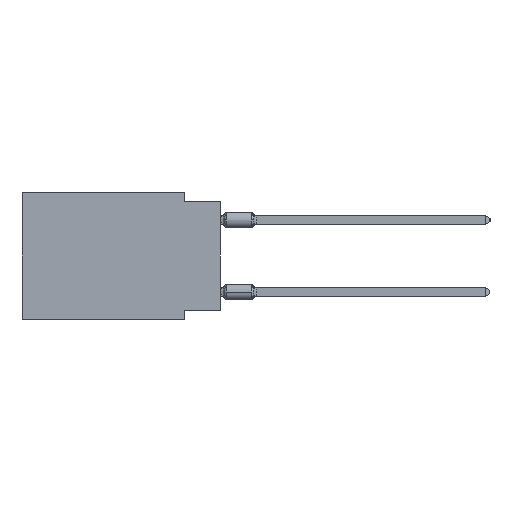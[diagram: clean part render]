
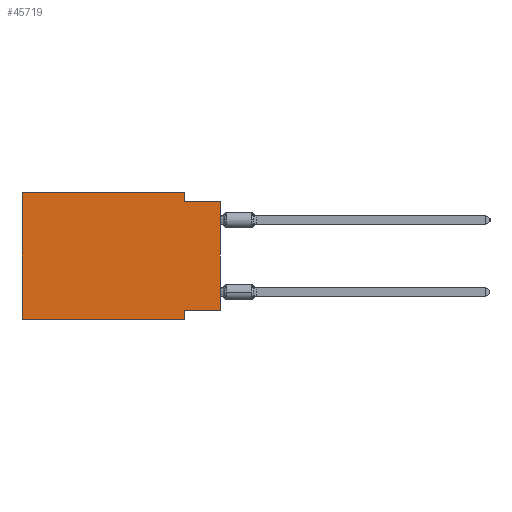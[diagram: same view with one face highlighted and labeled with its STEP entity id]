
A CAD part, left-side view. The second image highlights one B-rep face of the part: STEP entity #45719.
In plain terms, the highlighted planar face has unit normal (-1, 0, 0).
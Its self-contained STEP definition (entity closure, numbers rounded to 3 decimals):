
#1503 = CARTESIAN_POINT ( 'NONE',  ( 0., 13.97, -8.89 ) ) ;
#2421 = CARTESIAN_POINT ( 'NONE',  ( 0., 13.97, -8.89 ) ) ;
#2617 = CARTESIAN_POINT ( 'NONE',  ( 0., 2.54, 0. ) ) ;
#5274 = CARTESIAN_POINT ( 'NONE',  ( 0., 0., 0. ) ) ;
#5318 = VERTEX_POINT ( 'NONE', #34277 ) ;
#6966 = ORIENTED_EDGE ( 'NONE', *, *, #13096, .F. ) ;
#6985 = VECTOR ( 'NONE', #33532, 1000. ) ;
#7600 = DIRECTION ( 'NONE',  ( 0., 0., -1. ) ) ;
#7608 = LINE ( 'NONE', #27899, #28563 ) ;
#8690 = ORIENTED_EDGE ( 'NONE', *, *, #14452, .F. ) ;
#9925 = DIRECTION ( 'NONE',  ( 0., -1., 0. ) ) ;
#11632 = CARTESIAN_POINT ( 'NONE',  ( 0., 0., -8.255 ) ) ;
#12003 = CARTESIAN_POINT ( 'NONE',  ( 0., 13.97, 0. ) ) ;
#12917 = VERTEX_POINT ( 'NONE', #30679 ) ;
#13096 = EDGE_CURVE ( 'NONE', #50201, #5318, #27880, .T. ) ;
#13294 = EDGE_CURVE ( 'NONE', #20898, #40234, #38496, .T. ) ;
#13916 = ORIENTED_EDGE ( 'NONE', *, *, #34729, .T. ) ;
#14452 = EDGE_CURVE ( 'NONE', #28546, #12917, #22585, .T. ) ;
#15229 = VECTOR ( 'NONE', #26466, 1000. ) ;
#15240 = DIRECTION ( 'NONE',  ( 0., 0., 1. ) ) ;
#15717 = CARTESIAN_POINT ( 'NONE',  ( 0., 0., -0.635 ) ) ;
#20339 = EDGE_CURVE ( 'NONE', #20898, #51565, #46730, .T. ) ;
#20396 = CARTESIAN_POINT ( 'NONE',  ( 0., 0., -0.635 ) ) ;
#20777 = EDGE_CURVE ( 'NONE', #12917, #61230, #25393, .T. ) ;
#20898 = VERTEX_POINT ( 'NONE', #2421 ) ;
#21700 = CARTESIAN_POINT ( 'NONE',  ( 0., 2.54, -8.89 ) ) ;
#21777 = AXIS2_PLACEMENT_3D ( 'NONE', #12003, #42916, #57870 ) ;
#21846 = VECTOR ( 'NONE', #21936, 1000. ) ;
#21936 = DIRECTION ( 'NONE',  ( 0., 1., 0. ) ) ;
#22510 = EDGE_LOOP ( 'NONE', ( #13916, #53146, #8690, #54190, #54438, #48110, #46343, #6966 ) ) ;
#22585 = LINE ( 'NONE', #2617, #45269 ) ;
#24821 = VECTOR ( 'NONE', #40674, 1000. ) ;
#25393 = LINE ( 'NONE', #20396, #24821 ) ;
#26039 = EDGE_CURVE ( 'NONE', #40234, #28546, #61986, .T. ) ;
#26466 = DIRECTION ( 'NONE',  ( 0., -1., 0. ) ) ;
#26644 = PLANE ( 'NONE',  #21777 ) ;
#27454 = CARTESIAN_POINT ( 'NONE',  ( 0., 13.97, 0. ) ) ;
#27880 = LINE ( 'NONE', #11632, #21846 ) ;
#27899 = CARTESIAN_POINT ( 'NONE',  ( 0., 2.54, -8.89 ) ) ;
#28546 = VERTEX_POINT ( 'NONE', #43078 ) ;
#28563 = VECTOR ( 'NONE', #41873, 1000. ) ;
#30679 = CARTESIAN_POINT ( 'NONE',  ( 0., 2.54, -0.635 ) ) ;
#33532 = DIRECTION ( 'NONE',  ( 0., 0., 1. ) ) ;
#34277 = CARTESIAN_POINT ( 'NONE',  ( 0., 2.54, -8.255 ) ) ;
#34729 = EDGE_CURVE ( 'NONE', #50201, #61230, #39890, .T. ) ;
#38496 = LINE ( 'NONE', #60077, #6985 ) ;
#38591 = VECTOR ( 'NONE', #9925, 1000. ) ;
#39890 = LINE ( 'NONE', #5274, #59852 ) ;
#40005 = CARTESIAN_POINT ( 'NONE',  ( 0., 0., -8.255 ) ) ;
#40234 = VERTEX_POINT ( 'NONE', #51014 ) ;
#40674 = DIRECTION ( 'NONE',  ( 0., -1., 0. ) ) ;
#41873 = DIRECTION ( 'NONE',  ( 0., 0., -1. ) ) ;
#42916 = DIRECTION ( 'NONE',  ( 1., 0., 0. ) ) ;
#43078 = CARTESIAN_POINT ( 'NONE',  ( 0., 2.54, 0. ) ) ;
#45269 = VECTOR ( 'NONE', #7600, 1000. ) ;
#45719 = ADVANCED_FACE ( 'NONE', ( #63520 ), #26644, .F. ) ;
#46343 = ORIENTED_EDGE ( 'NONE', *, *, #50887, .F. ) ;
#46730 = LINE ( 'NONE', #1503, #38591 ) ;
#48110 = ORIENTED_EDGE ( 'NONE', *, *, #20339, .T. ) ;
#50201 = VERTEX_POINT ( 'NONE', #40005 ) ;
#50887 = EDGE_CURVE ( 'NONE', #5318, #51565, #7608, .T. ) ;
#51014 = CARTESIAN_POINT ( 'NONE',  ( 0., 13.97, 0. ) ) ;
#51565 = VERTEX_POINT ( 'NONE', #21700 ) ;
#53146 = ORIENTED_EDGE ( 'NONE', *, *, #20777, .F. ) ;
#54190 = ORIENTED_EDGE ( 'NONE', *, *, #26039, .F. ) ;
#54438 = ORIENTED_EDGE ( 'NONE', *, *, #13294, .F. ) ;
#57870 = DIRECTION ( 'NONE',  ( 0., 0., -1. ) ) ;
#59852 = VECTOR ( 'NONE', #15240, 1000. ) ;
#60077 = CARTESIAN_POINT ( 'NONE',  ( 0., 13.97, 0. ) ) ;
#61230 = VERTEX_POINT ( 'NONE', #15717 ) ;
#61986 = LINE ( 'NONE', #27454, #15229 ) ;
#63520 = FACE_OUTER_BOUND ( 'NONE', #22510, .T. ) ;
